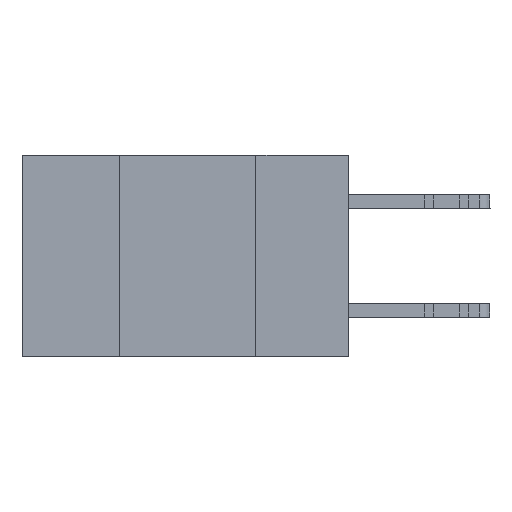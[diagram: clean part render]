
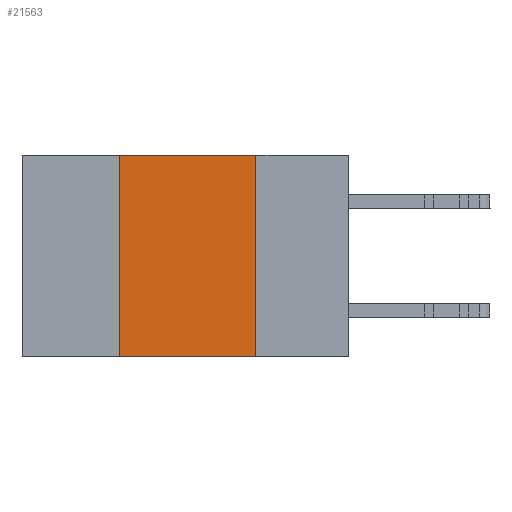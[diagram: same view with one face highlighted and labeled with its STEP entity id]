
A CAD part, left-side view. The second image highlights one B-rep face of the part: STEP entity #21563.
In plain terms, the highlighted planar face has unit normal (-1, 0, 0).
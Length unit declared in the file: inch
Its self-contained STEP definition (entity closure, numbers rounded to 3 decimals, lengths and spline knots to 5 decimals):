
#2267 = AXIS2_PLACEMENT_3D ( 'NONE', #16330, #3067, #18595 ) ;
#2340 = VECTOR ( 'NONE', #23217, 39.37008 ) ;
#2684 = CARTESIAN_POINT ( 'NONE',  ( 0., 0.17, 0. ) ) ;
#2814 = EDGE_CURVE ( 'NONE', #15468, #7753, #13452, .T. ) ;
#3067 = DIRECTION ( 'NONE',  ( 1., 0., 0. ) ) ;
#3766 = VERTEX_POINT ( 'NONE', #2684 ) ;
#4452 = LINE ( 'NONE', #8430, #15504 ) ;
#4864 = DIRECTION ( 'NONE',  ( 0., 0., 1. ) ) ;
#5354 = VECTOR ( 'NONE', #17391, 39.37008 ) ;
#6024 = LINE ( 'NONE', #15163, #5354 ) ;
#7463 = CARTESIAN_POINT ( 'NONE',  ( 0., 0.6, -0.37 ) ) ;
#7753 = VERTEX_POINT ( 'NONE', #22090 ) ;
#7793 = LINE ( 'NONE', #18100, #19512 ) ;
#7817 = ORIENTED_EDGE ( 'NONE', *, *, #21421, .F. ) ;
#8430 = CARTESIAN_POINT ( 'NONE',  ( 0., 0.17, 0. ) ) ;
#8673 = ORIENTED_EDGE ( 'NONE', *, *, #2814, .T. ) ;
#10200 = FACE_OUTER_BOUND ( 'NONE', #21710, .T. ) ;
#12438 = ORIENTED_EDGE ( 'NONE', *, *, #12682, .F. ) ;
#12682 = EDGE_CURVE ( 'NONE', #21398, #3766, #6024, .T. ) ;
#13292 = ORIENTED_EDGE ( 'NONE', *, *, #24396, .F. ) ;
#13452 = LINE ( 'NONE', #7463, #2340 ) ;
#15163 = CARTESIAN_POINT ( 'NONE',  ( 0., 0.6, 0. ) ) ;
#15468 = VERTEX_POINT ( 'NONE', #23406 ) ;
#15504 = VECTOR ( 'NONE', #19434, 39.37008 ) ;
#16330 = CARTESIAN_POINT ( 'NONE',  ( 0., 0.6, 0. ) ) ;
#17391 = DIRECTION ( 'NONE',  ( 0., -1., 0. ) ) ;
#17995 = CARTESIAN_POINT ( 'NONE',  ( 0., 0.42, 0. ) ) ;
#18100 = CARTESIAN_POINT ( 'NONE',  ( 0., 0.42, 0. ) ) ;
#18595 = DIRECTION ( 'NONE',  ( 0., 0., -1. ) ) ;
#19434 = DIRECTION ( 'NONE',  ( 0., 0., -1. ) ) ;
#19512 = VECTOR ( 'NONE', #4864, 39.37008 ) ;
#20726 = PLANE ( 'NONE',  #2267 ) ;
#21398 = VERTEX_POINT ( 'NONE', #17995 ) ;
#21421 = EDGE_CURVE ( 'NONE', #15468, #21398, #7793, .T. ) ;
#21563 = ADVANCED_FACE ( 'NONE', ( #10200 ), #20726, .F. ) ;
#21710 = EDGE_LOOP ( 'NONE', ( #13292, #12438, #7817, #8673 ) ) ;
#22090 = CARTESIAN_POINT ( 'NONE',  ( 0., 0.17, -0.37 ) ) ;
#23217 = DIRECTION ( 'NONE',  ( 0., -1., 0. ) ) ;
#23406 = CARTESIAN_POINT ( 'NONE',  ( 0., 0.42, -0.37 ) ) ;
#24396 = EDGE_CURVE ( 'NONE', #3766, #7753, #4452, .T. ) ;
